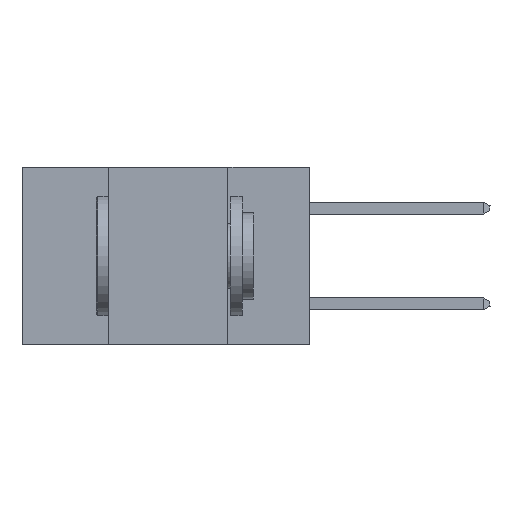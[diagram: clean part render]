
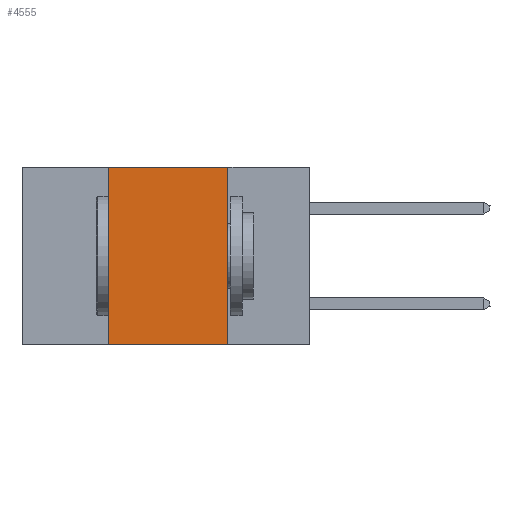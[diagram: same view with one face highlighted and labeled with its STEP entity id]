
A CAD part, left-side view. The second image highlights one B-rep face of the part: STEP entity #4555.
In plain terms, the highlighted planar face has unit normal (-1, 0, 0).
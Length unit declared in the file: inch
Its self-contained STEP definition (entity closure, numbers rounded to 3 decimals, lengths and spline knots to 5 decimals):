
#716 = PLANE ( 'NONE',  #11101 ) ;
#732 = LINE ( 'NONE', #17013, #7355 ) ;
#882 = VERTEX_POINT ( 'NONE', #7488 ) ;
#1040 = LINE ( 'NONE', #13486, #2876 ) ;
#1441 = EDGE_CURVE ( 'NONE', #882, #17338, #7651, .T. ) ;
#1707 = ORIENTED_EDGE ( 'NONE', *, *, #6582, .F. ) ;
#1739 = VECTOR ( 'NONE', #10078, 39.37008 ) ;
#2876 = VECTOR ( 'NONE', #11956, 39.37008 ) ;
#3271 = VECTOR ( 'NONE', #12037, 39.37008 ) ;
#3516 = EDGE_CURVE ( 'NONE', #17338, #13092, #1040, .T. ) ;
#4401 = LINE ( 'NONE', #16400, #3271 ) ;
#4555 = ADVANCED_FACE ( 'NONE', ( #17395 ), #716, .F. ) ;
#5113 = CARTESIAN_POINT ( 'NONE',  ( 0., 0.6, 0. ) ) ;
#5371 = EDGE_LOOP ( 'NONE', ( #12180, #15214, #1707, #18735 ) ) ;
#5813 = EDGE_CURVE ( 'NONE', #15514, #13092, #4401, .T. ) ;
#5845 = CARTESIAN_POINT ( 'NONE',  ( 0., 0.17, 0. ) ) ;
#6582 = EDGE_CURVE ( 'NONE', #15514, #882, #732, .T. ) ;
#7355 = VECTOR ( 'NONE', #18405, 39.37008 ) ;
#7488 = CARTESIAN_POINT ( 'NONE',  ( 0., 0.42, 0. ) ) ;
#7651 = LINE ( 'NONE', #17149, #1739 ) ;
#10078 = DIRECTION ( 'NONE',  ( 0., -1., 0. ) ) ;
#11101 = AXIS2_PLACEMENT_3D ( 'NONE', #5113, #13901, #16789 ) ;
#11956 = DIRECTION ( 'NONE',  ( 0., 0., -1. ) ) ;
#12037 = DIRECTION ( 'NONE',  ( 0., -1., 0. ) ) ;
#12180 = ORIENTED_EDGE ( 'NONE', *, *, #3516, .F. ) ;
#13092 = VERTEX_POINT ( 'NONE', #18333 ) ;
#13486 = CARTESIAN_POINT ( 'NONE',  ( 0., 0.17, 0. ) ) ;
#13901 = DIRECTION ( 'NONE',  ( 1., 0., 0. ) ) ;
#15214 = ORIENTED_EDGE ( 'NONE', *, *, #1441, .F. ) ;
#15514 = VERTEX_POINT ( 'NONE', #17444 ) ;
#16400 = CARTESIAN_POINT ( 'NONE',  ( 0., 0.6, -0.37 ) ) ;
#16789 = DIRECTION ( 'NONE',  ( 0., 0., -1. ) ) ;
#17013 = CARTESIAN_POINT ( 'NONE',  ( 0., 0.42, 0. ) ) ;
#17149 = CARTESIAN_POINT ( 'NONE',  ( 0., 0.6, 0. ) ) ;
#17338 = VERTEX_POINT ( 'NONE', #5845 ) ;
#17395 = FACE_OUTER_BOUND ( 'NONE', #5371, .T. ) ;
#17444 = CARTESIAN_POINT ( 'NONE',  ( 0., 0.42, -0.37 ) ) ;
#18333 = CARTESIAN_POINT ( 'NONE',  ( 0., 0.17, -0.37 ) ) ;
#18405 = DIRECTION ( 'NONE',  ( 0., 0., 1. ) ) ;
#18735 = ORIENTED_EDGE ( 'NONE', *, *, #5813, .T. ) ;
